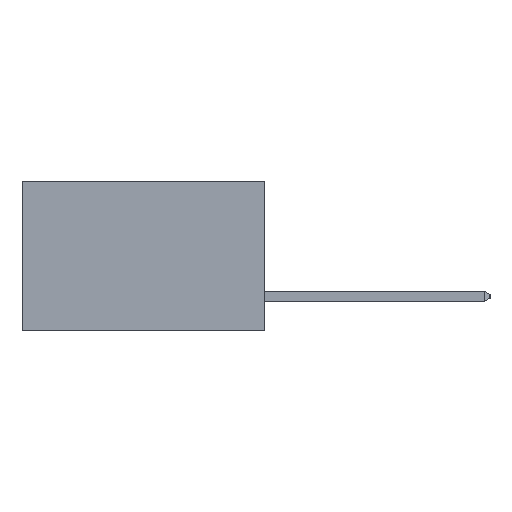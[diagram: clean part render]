
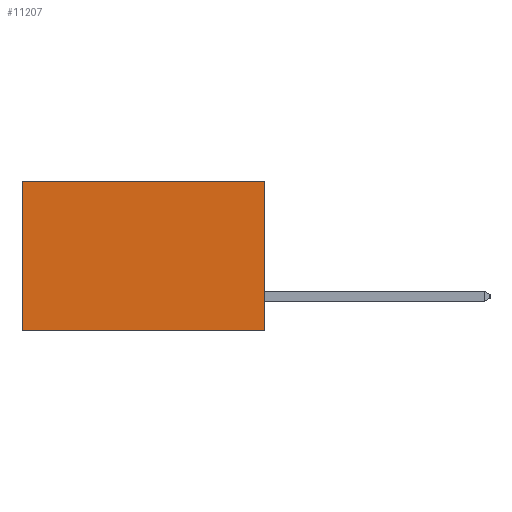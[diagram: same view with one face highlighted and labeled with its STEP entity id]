
A CAD part, left-side view. The second image highlights one B-rep face of the part: STEP entity #11207.
In plain terms, the highlighted planar face has unit normal (-1, 0, 0).
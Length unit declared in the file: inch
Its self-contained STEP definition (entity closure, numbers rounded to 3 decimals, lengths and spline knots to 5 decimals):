
#394 = EDGE_CURVE ( 'NONE', #8614, #17756, #15394, .T. ) ;
#786 = LINE ( 'NONE', #1170, #4827 ) ;
#917 = ORIENTED_EDGE ( 'NONE', *, *, #4393, .T. ) ;
#1170 = CARTESIAN_POINT ( 'NONE',  ( 0.2615, 0.6, -0.37 ) ) ;
#3916 = LINE ( 'NONE', #18105, #15771 ) ;
#4250 = VERTEX_POINT ( 'NONE', #8951 ) ;
#4393 = EDGE_CURVE ( 'NONE', #4250, #14018, #11387, .T. ) ;
#4827 = VECTOR ( 'NONE', #10238, 39.37008 ) ;
#5351 = CARTESIAN_POINT ( 'NONE',  ( 0.2615, 0.6, -0.37 ) ) ;
#6384 = CARTESIAN_POINT ( 'NONE',  ( 0.2615, 0., 0. ) ) ;
#6502 = DIRECTION ( 'NONE',  ( 0., 1., 0. ) ) ;
#6556 = FACE_OUTER_BOUND ( 'NONE', #16809, .T. ) ;
#8039 = PLANE ( 'NONE',  #18025 ) ;
#8614 = VERTEX_POINT ( 'NONE', #9713 ) ;
#8951 = CARTESIAN_POINT ( 'NONE',  ( 0.2615, 0., 0. ) ) ;
#9476 = CARTESIAN_POINT ( 'NONE',  ( 0.2615, 0., -0.37 ) ) ;
#9539 = DIRECTION ( 'NONE',  ( 0., 0., -1. ) ) ;
#9713 = CARTESIAN_POINT ( 'NONE',  ( 0.2615, 0., -0.37 ) ) ;
#10238 = DIRECTION ( 'NONE',  ( 0., 0., -1. ) ) ;
#11207 = ADVANCED_FACE ( 'NONE', ( #6556 ), #8039, .F. ) ;
#11387 = LINE ( 'NONE', #6384, #18990 ) ;
#12420 = EDGE_CURVE ( 'NONE', #4250, #8614, #3916, .T. ) ;
#12932 = ORIENTED_EDGE ( 'NONE', *, *, #12420, .F. ) ;
#12991 = EDGE_CURVE ( 'NONE', #14018, #17756, #786, .T. ) ;
#13224 = DIRECTION ( 'NONE',  ( 0., 1., 0. ) ) ;
#13738 = ORIENTED_EDGE ( 'NONE', *, *, #12991, .T. ) ;
#14018 = VERTEX_POINT ( 'NONE', #17385 ) ;
#14916 = VECTOR ( 'NONE', #13224, 39.37008 ) ;
#15394 = LINE ( 'NONE', #17724, #14916 ) ;
#15771 = VECTOR ( 'NONE', #19573, 39.37008 ) ;
#16809 = EDGE_LOOP ( 'NONE', ( #13738, #18316, #12932, #917 ) ) ;
#17385 = CARTESIAN_POINT ( 'NONE',  ( 0.2615, 0.6, 0. ) ) ;
#17724 = CARTESIAN_POINT ( 'NONE',  ( 0.2615, 0., -0.37 ) ) ;
#17756 = VERTEX_POINT ( 'NONE', #5351 ) ;
#18025 = AXIS2_PLACEMENT_3D ( 'NONE', #9476, #18656, #9539 ) ;
#18105 = CARTESIAN_POINT ( 'NONE',  ( 0.2615, 0., -0.37 ) ) ;
#18316 = ORIENTED_EDGE ( 'NONE', *, *, #394, .F. ) ;
#18656 = DIRECTION ( 'NONE',  ( 1., 0., 0. ) ) ;
#18990 = VECTOR ( 'NONE', #6502, 39.37008 ) ;
#19573 = DIRECTION ( 'NONE',  ( 0., 0., -1. ) ) ;
